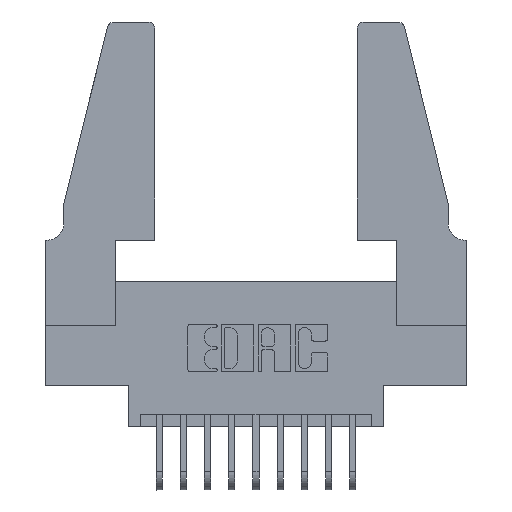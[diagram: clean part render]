
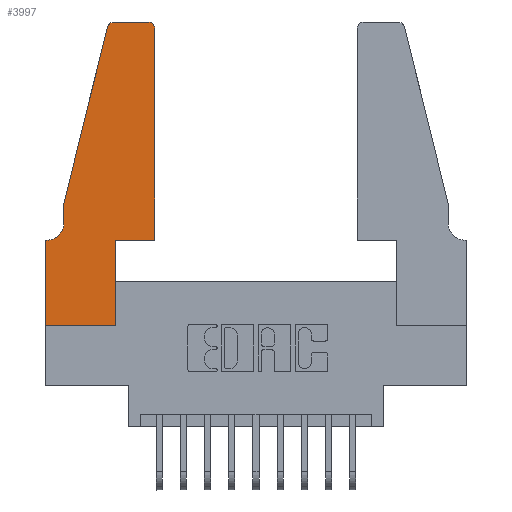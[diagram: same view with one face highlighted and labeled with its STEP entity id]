
A CAD part, top view. The second image highlights one B-rep face of the part: STEP entity #3997.
In plain terms, the highlighted planar face has unit normal (0, 0, 1).
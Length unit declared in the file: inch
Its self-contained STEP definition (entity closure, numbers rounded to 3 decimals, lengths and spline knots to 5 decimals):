
#153 = VERTEX_POINT ( 'NONE', #12569 ) ;
#290 = EDGE_CURVE ( 'NONE', #2160, #7784, #12773, .T. ) ;
#333 = VERTEX_POINT ( 'NONE', #2888 ) ;
#586 = VECTOR ( 'NONE', #10907, 39.37008 ) ;
#931 = LINE ( 'NONE', #9997, #586 ) ;
#1071 = EDGE_CURVE ( 'NONE', #6939, #1938, #931, .T. ) ;
#1149 = EDGE_CURVE ( 'NONE', #333, #7691, #12896, .T. ) ;
#1370 = LINE ( 'NONE', #3514, #12228 ) ;
#1493 = EDGE_CURVE ( 'NONE', #7784, #333, #5239, .T. ) ;
#1584 = ORIENTED_EDGE ( 'NONE', *, *, #11846, .T. ) ;
#1720 = DIRECTION ( 'NONE',  ( -0.239, -0.971, 0. ) ) ;
#1938 = VERTEX_POINT ( 'NONE', #5860 ) ;
#2046 = EDGE_CURVE ( 'NONE', #3718, #153, #9977, .T. ) ;
#2160 = VERTEX_POINT ( 'NONE', #9359 ) ;
#2217 = AXIS2_PLACEMENT_3D ( 'NONE', #11029, #11079, #4919 ) ;
#2357 = AXIS2_PLACEMENT_3D ( 'NONE', #6042, #5861, #5798 ) ;
#2358 = ORIENTED_EDGE ( 'NONE', *, *, #5935, .T. ) ;
#2576 = ORIENTED_EDGE ( 'NONE', *, *, #1071, .T. ) ;
#2578 = VERTEX_POINT ( 'NONE', #3801 ) ;
#2888 = CARTESIAN_POINT ( 'NONE',  ( 0.0755, 0.42, 0.37 ) ) ;
#3163 = ORIENTED_EDGE ( 'NONE', *, *, #1149, .T. ) ;
#3256 = LINE ( 'NONE', #13215, #8448 ) ;
#3300 = VERTEX_POINT ( 'NONE', #4034 ) ;
#3385 = ORIENTED_EDGE ( 'NONE', *, *, #4971, .T. ) ;
#3427 = ORIENTED_EDGE ( 'NONE', *, *, #13496, .T. ) ;
#3514 = CARTESIAN_POINT ( 'NONE',  ( 0., 0., 0.37 ) ) ;
#3620 = ORIENTED_EDGE ( 'NONE', *, *, #2046, .T. ) ;
#3638 = ORIENTED_EDGE ( 'NONE', *, *, #9226, .T. ) ;
#3718 = VERTEX_POINT ( 'NONE', #9043 ) ;
#3801 = CARTESIAN_POINT ( 'NONE',  ( 0.4205, 1.25, 0.37 ) ) ;
#3813 = DIRECTION ( 'NONE',  ( 1., 0., 0. ) ) ;
#3997 = ADVANCED_FACE ( 'NONE', ( #5353 ), #5929, .T. ) ;
#4034 = CARTESIAN_POINT ( 'NONE',  ( 0., 0.35, 0.37 ) ) ;
#4178 = CARTESIAN_POINT ( 'NONE',  ( 0.4205, 1.22, 0.37 ) ) ;
#4291 = CARTESIAN_POINT ( 'NONE',  ( 0.284, 1.25, 0.37 ) ) ;
#4838 = CARTESIAN_POINT ( 'NONE',  ( 0.284, 1.22, 0.37 ) ) ;
#4919 = DIRECTION ( 'NONE',  ( 1., 0., 0. ) ) ;
#4971 = EDGE_CURVE ( 'NONE', #5644, #3718, #6261, .T. ) ;
#5123 = VECTOR ( 'NONE', #11515, 39.37008 ) ;
#5239 = LINE ( 'NONE', #13309, #8237 ) ;
#5257 = DIRECTION ( 'NONE',  ( 1., 0., 0. ) ) ;
#5353 = FACE_OUTER_BOUND ( 'NONE', #9789, .T. ) ;
#5574 = EDGE_CURVE ( 'NONE', #7980, #2160, #8285, .T. ) ;
#5644 = VERTEX_POINT ( 'NONE', #11125 ) ;
#5798 = DIRECTION ( 'NONE',  ( -1., 0., 0. ) ) ;
#5860 = CARTESIAN_POINT ( 'NONE',  ( 0.4505, 1.22, 0.37 ) ) ;
#5861 = DIRECTION ( 'NONE',  ( 0., 0., -1. ) ) ;
#5888 = DIRECTION ( 'NONE',  ( 1., 0., 0. ) ) ;
#5929 = PLANE ( 'NONE',  #2217 ) ;
#5935 = EDGE_CURVE ( 'NONE', #153, #6939, #12323, .T. ) ;
#6042 = CARTESIAN_POINT ( 'NONE',  ( 0.0055, 0.42, 0.37 ) ) ;
#6100 = DIRECTION ( 'NONE',  ( -1., 0., 0. ) ) ;
#6190 = DIRECTION ( 'NONE',  ( 0., -1., 0. ) ) ;
#6261 = LINE ( 'NONE', #11046, #8959 ) ;
#6566 = EDGE_CURVE ( 'NONE', #2578, #7980, #9870, .T. ) ;
#6939 = VERTEX_POINT ( 'NONE', #9998 ) ;
#6955 = VECTOR ( 'NONE', #7083, 39.37008 ) ;
#7001 = ORIENTED_EDGE ( 'NONE', *, *, #5574, .T. ) ;
#7083 = DIRECTION ( 'NONE',  ( 0., 1., 0. ) ) ;
#7679 = DIRECTION ( 'NONE',  ( 0., -1., 0. ) ) ;
#7691 = VERTEX_POINT ( 'NONE', #8012 ) ;
#7784 = VERTEX_POINT ( 'NONE', #8099 ) ;
#7980 = VERTEX_POINT ( 'NONE', #4291 ) ;
#8012 = CARTESIAN_POINT ( 'NONE',  ( 0.0055, 0.35, 0.37 ) ) ;
#8099 = CARTESIAN_POINT ( 'NONE',  ( 0.0755, 0.5, 0.37 ) ) ;
#8237 = VECTOR ( 'NONE', #6190, 39.37008 ) ;
#8285 = CIRCLE ( 'NONE', #13193, 0.03 ) ;
#8448 = VECTOR ( 'NONE', #6100, 39.37008 ) ;
#8546 = AXIS2_PLACEMENT_3D ( 'NONE', #4178, #11391, #5257 ) ;
#8959 = VECTOR ( 'NONE', #3813, 39.37008 ) ;
#9043 = CARTESIAN_POINT ( 'NONE',  ( 0.2865, 0., 0.37 ) ) ;
#9226 = EDGE_CURVE ( 'NONE', #1938, #2578, #12130, .T. ) ;
#9359 = CARTESIAN_POINT ( 'NONE',  ( 0.25487, 1.22718, 0.37 ) ) ;
#9400 = ORIENTED_EDGE ( 'NONE', *, *, #6566, .T. ) ;
#9708 = ORIENTED_EDGE ( 'NONE', *, *, #290, .T. ) ;
#9789 = EDGE_LOOP ( 'NONE', ( #9400, #7001, #9708, #12769, #3163, #3427, #1584, #3385, #3620, #2358, #2576, #3638 ) ) ;
#9870 = LINE ( 'NONE', #12345, #12311 ) ;
#9977 = LINE ( 'NONE', #12215, #6955 ) ;
#9997 = CARTESIAN_POINT ( 'NONE',  ( 0.4505, 0.35, 0.37 ) ) ;
#9998 = CARTESIAN_POINT ( 'NONE',  ( 0.4505, 0.35, 0.37 ) ) ;
#10039 = VECTOR ( 'NONE', #1720, 39.37008 ) ;
#10907 = DIRECTION ( 'NONE',  ( 0., 1., 0. ) ) ;
#11029 = CARTESIAN_POINT ( 'NONE',  ( 0., 0.35, 0.37 ) ) ;
#11046 = CARTESIAN_POINT ( 'NONE',  ( 0., 0., 0.37 ) ) ;
#11079 = DIRECTION ( 'NONE',  ( 0., 0., 1. ) ) ;
#11125 = CARTESIAN_POINT ( 'NONE',  ( 0., 0., 0.37 ) ) ;
#11138 = CARTESIAN_POINT ( 'NONE',  ( 0.0755, 0.5, 0.37 ) ) ;
#11391 = DIRECTION ( 'NONE',  ( 0., 0., 1. ) ) ;
#11515 = DIRECTION ( 'NONE',  ( 1., 0., 0. ) ) ;
#11567 = CARTESIAN_POINT ( 'NONE',  ( 0.4505, 0.35, 0.37 ) ) ;
#11846 = EDGE_CURVE ( 'NONE', #3300, #5644, #1370, .T. ) ;
#12008 = DIRECTION ( 'NONE',  ( 0., 0., 1. ) ) ;
#12130 = CIRCLE ( 'NONE', #8546, 0.03 ) ;
#12215 = CARTESIAN_POINT ( 'NONE',  ( 0.2865, 0.35, 0.37 ) ) ;
#12228 = VECTOR ( 'NONE', #7679, 39.37008 ) ;
#12311 = VECTOR ( 'NONE', #13340, 39.37008 ) ;
#12323 = LINE ( 'NONE', #11567, #5123 ) ;
#12345 = CARTESIAN_POINT ( 'NONE',  ( 0.2605, 1.25, 0.37 ) ) ;
#12569 = CARTESIAN_POINT ( 'NONE',  ( 0.2865, 0.35, 0.37 ) ) ;
#12769 = ORIENTED_EDGE ( 'NONE', *, *, #1493, .T. ) ;
#12773 = LINE ( 'NONE', #11138, #10039 ) ;
#12896 = CIRCLE ( 'NONE', #2357, 0.07 ) ;
#13193 = AXIS2_PLACEMENT_3D ( 'NONE', #4838, #12008, #5888 ) ;
#13215 = CARTESIAN_POINT ( 'NONE',  ( 0.0755, 0.35, 0.37 ) ) ;
#13309 = CARTESIAN_POINT ( 'NONE',  ( 0.0755, 0.5, 0.37 ) ) ;
#13340 = DIRECTION ( 'NONE',  ( -1., 0., 0. ) ) ;
#13496 = EDGE_CURVE ( 'NONE', #7691, #3300, #3256, .T. ) ;
